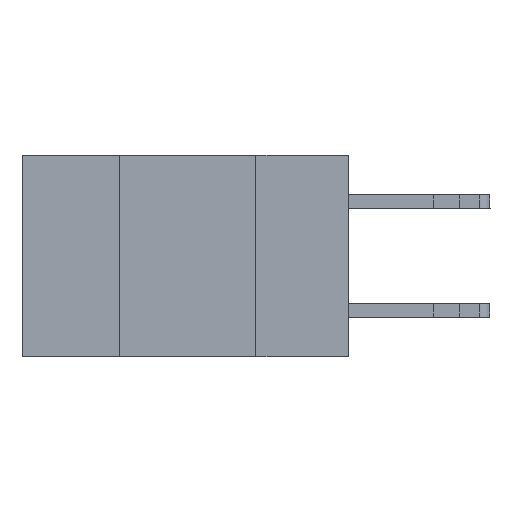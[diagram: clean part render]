
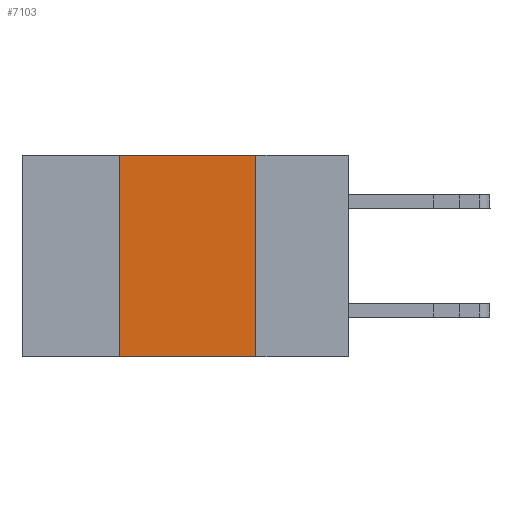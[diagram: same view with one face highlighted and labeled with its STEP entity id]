
A CAD part, left-side view. The second image highlights one B-rep face of the part: STEP entity #7103.
In plain terms, the highlighted planar face has unit normal (-1, 0, 0).
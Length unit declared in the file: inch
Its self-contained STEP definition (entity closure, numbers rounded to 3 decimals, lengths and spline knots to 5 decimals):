
#173 = VERTEX_POINT ( 'NONE', #19966 ) ;
#1363 = LINE ( 'NONE', #19722, #10701 ) ;
#2068 = ORIENTED_EDGE ( 'NONE', *, *, #14444, .T. ) ;
#2099 = ORIENTED_EDGE ( 'NONE', *, *, #10678, .F. ) ;
#2113 = CARTESIAN_POINT ( 'NONE',  ( 0., 0.42, -0.37 ) ) ;
#2720 = CARTESIAN_POINT ( 'NONE',  ( 0., 0.6, 0. ) ) ;
#3841 = CARTESIAN_POINT ( 'NONE',  ( 0., 0.17, 0. ) ) ;
#4006 = PLANE ( 'NONE',  #18277 ) ;
#5348 = ORIENTED_EDGE ( 'NONE', *, *, #12483, .F. ) ;
#5634 = FACE_OUTER_BOUND ( 'NONE', #14509, .T. ) ;
#5743 = EDGE_CURVE ( 'NONE', #21175, #15793, #11738, .T. ) ;
#5757 = DIRECTION ( 'NONE',  ( 0., -1., 0. ) ) ;
#6380 = VERTEX_POINT ( 'NONE', #2113 ) ;
#7103 = ADVANCED_FACE ( 'NONE', ( #5634 ), #4006, .F. ) ;
#8950 = CARTESIAN_POINT ( 'NONE',  ( 0., 0.42, -0.37 ) ) ;
#10286 = ORIENTED_EDGE ( 'NONE', *, *, #5743, .F. ) ;
#10528 = LINE ( 'NONE', #2720, #14452 ) ;
#10630 = CARTESIAN_POINT ( 'NONE',  ( 0., 0.6, 0. ) ) ;
#10678 = EDGE_CURVE ( 'NONE', #6380, #173, #12328, .T. ) ;
#10701 = VECTOR ( 'NONE', #17985, 39.37008 ) ;
#11738 = LINE ( 'NONE', #16288, #19625 ) ;
#11981 = CARTESIAN_POINT ( 'NONE',  ( 0., 0.17, -0.37 ) ) ;
#12328 = LINE ( 'NONE', #8950, #20307 ) ;
#12483 = EDGE_CURVE ( 'NONE', #173, #21175, #10528, .T. ) ;
#14401 = DIRECTION ( 'NONE',  ( 1., 0., 0. ) ) ;
#14444 = EDGE_CURVE ( 'NONE', #6380, #15793, #1363, .T. ) ;
#14452 = VECTOR ( 'NONE', #5757, 39.37008 ) ;
#14509 = EDGE_LOOP ( 'NONE', ( #10286, #5348, #2099, #2068 ) ) ;
#15793 = VERTEX_POINT ( 'NONE', #11981 ) ;
#16288 = CARTESIAN_POINT ( 'NONE',  ( 0., 0.17, -0.37 ) ) ;
#17521 = DIRECTION ( 'NONE',  ( 0., 0., 1. ) ) ;
#17985 = DIRECTION ( 'NONE',  ( 0., -1., 0. ) ) ;
#18277 = AXIS2_PLACEMENT_3D ( 'NONE', #10630, #14401, #21361 ) ;
#19625 = VECTOR ( 'NONE', #19772, 39.37008 ) ;
#19722 = CARTESIAN_POINT ( 'NONE',  ( 0., 0.6, -0.37 ) ) ;
#19772 = DIRECTION ( 'NONE',  ( 0., 0., -1. ) ) ;
#19966 = CARTESIAN_POINT ( 'NONE',  ( 0., 0.42, 0. ) ) ;
#20307 = VECTOR ( 'NONE', #17521, 39.37008 ) ;
#21175 = VERTEX_POINT ( 'NONE', #3841 ) ;
#21361 = DIRECTION ( 'NONE',  ( 0., 0., -1. ) ) ;
